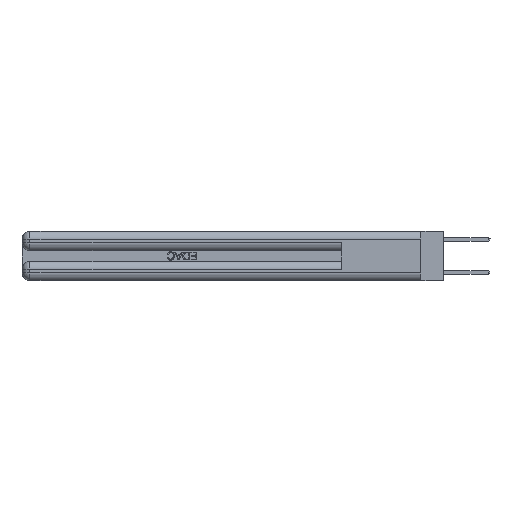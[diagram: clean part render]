
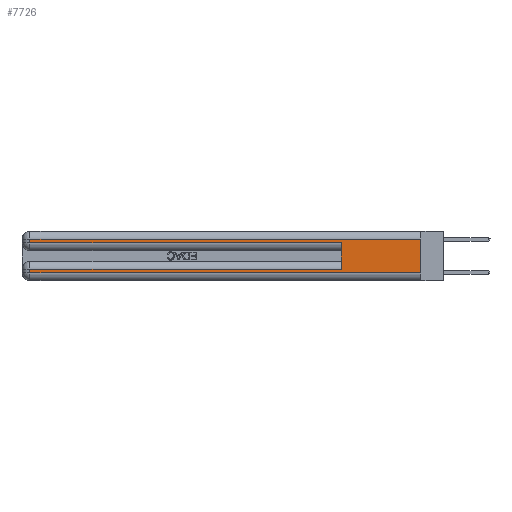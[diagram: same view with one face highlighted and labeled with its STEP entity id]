
A CAD part, left-side view. The second image highlights one B-rep face of the part: STEP entity #7726.
In plain terms, the highlighted planar face has unit normal (-1, 0, 0).
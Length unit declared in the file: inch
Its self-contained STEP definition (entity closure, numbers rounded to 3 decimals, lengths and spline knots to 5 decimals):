
#483 = DIRECTION ( 'NONE',  ( 1., 0., 0. ) ) ;
#1186 = PLANE ( 'NONE',  #19913 ) ;
#1325 = CARTESIAN_POINT ( 'NONE',  ( 0., 0., 0.31 ) ) ;
#2356 = LINE ( 'NONE', #18788, #3348 ) ;
#3005 = LINE ( 'NONE', #22045, #14640 ) ;
#3050 = LINE ( 'NONE', #23939, #21876 ) ;
#3135 = CARTESIAN_POINT ( 'NONE',  ( 0., 0.6, 0.285 ) ) ;
#3348 = VECTOR ( 'NONE', #11640, 39.37008 ) ;
#4142 = DIRECTION ( 'NONE',  ( 0., 0., -1. ) ) ;
#4411 = CARTESIAN_POINT ( 'NONE',  ( 0., 0., 0.37 ) ) ;
#4921 = ORIENTED_EDGE ( 'NONE', *, *, #17834, .T. ) ;
#5814 = VECTOR ( 'NONE', #25473, 39.37008 ) ;
#5973 = ORIENTED_EDGE ( 'NONE', *, *, #6416, .T. ) ;
#6234 = VECTOR ( 'NONE', #20308, 39.37008 ) ;
#6296 = CARTESIAN_POINT ( 'NONE',  ( 0., 2.94, 0.37 ) ) ;
#6416 = EDGE_CURVE ( 'NONE', #10710, #29371, #3005, .T. ) ;
#6460 = VERTEX_POINT ( 'NONE', #1325 ) ;
#7179 = CARTESIAN_POINT ( 'NONE',  ( 0., 0., 0.285 ) ) ;
#7595 = EDGE_CURVE ( 'NONE', #6460, #29371, #25033, .T. ) ;
#7726 = ADVANCED_FACE ( 'NONE', ( #14179 ), #1186, .F. ) ;
#8183 = CARTESIAN_POINT ( 'NONE',  ( 0., 2.94, 0.06 ) ) ;
#8397 = ORIENTED_EDGE ( 'NONE', *, *, #13000, .T. ) ;
#9335 = ORIENTED_EDGE ( 'NONE', *, *, #21855, .T. ) ;
#9799 = ORIENTED_EDGE ( 'NONE', *, *, #25341, .T. ) ;
#10225 = VERTEX_POINT ( 'NONE', #24566 ) ;
#10710 = VERTEX_POINT ( 'NONE', #8183 ) ;
#11241 = EDGE_CURVE ( 'NONE', #28706, #28387, #23354, .T. ) ;
#11640 = DIRECTION ( 'NONE',  ( 0., 1., 0. ) ) ;
#12295 = DIRECTION ( 'NONE',  ( 0., -1., 0. ) ) ;
#12493 = DIRECTION ( 'NONE',  ( 0., 0., 1. ) ) ;
#13000 = EDGE_CURVE ( 'NONE', #21127, #28706, #13157, .T. ) ;
#13157 = LINE ( 'NONE', #6296, #6234 ) ;
#13592 = EDGE_CURVE ( 'NONE', #24316, #28387, #3050, .T. ) ;
#14179 = FACE_OUTER_BOUND ( 'NONE', #17587, .T. ) ;
#14640 = VECTOR ( 'NONE', #12295, 39.37008 ) ;
#15031 = CARTESIAN_POINT ( 'NONE',  ( 0., 0., 0.085 ) ) ;
#16512 = CARTESIAN_POINT ( 'NONE',  ( 0., 2.94, 0.285 ) ) ;
#17587 = EDGE_LOOP ( 'NONE', ( #24046, #4921, #8397, #23573, #21399, #9799, #9335, #5973 ) ) ;
#17834 = EDGE_CURVE ( 'NONE', #6460, #21127, #2356, .T. ) ;
#17911 = VECTOR ( 'NONE', #24504, 39.37008 ) ;
#18309 = CARTESIAN_POINT ( 'NONE',  ( 0., 2.94, 0.37 ) ) ;
#18788 = CARTESIAN_POINT ( 'NONE',  ( 0., 0., 0.31 ) ) ;
#19913 = AXIS2_PLACEMENT_3D ( 'NONE', #25780, #483, #23935 ) ;
#20308 = DIRECTION ( 'NONE',  ( 0., 0., -1. ) ) ;
#20597 = DIRECTION ( 'NONE',  ( 0., -1., 0. ) ) ;
#21127 = VERTEX_POINT ( 'NONE', #28053 ) ;
#21399 = ORIENTED_EDGE ( 'NONE', *, *, #13592, .F. ) ;
#21855 = EDGE_CURVE ( 'NONE', #10225, #10710, #25355, .T. ) ;
#21876 = VECTOR ( 'NONE', #12493, 39.37008 ) ;
#22045 = CARTESIAN_POINT ( 'NONE',  ( 0., 0., 0.06 ) ) ;
#23354 = LINE ( 'NONE', #7179, #24624 ) ;
#23573 = ORIENTED_EDGE ( 'NONE', *, *, #11241, .T. ) ;
#23935 = DIRECTION ( 'NONE',  ( 0., 0., -1. ) ) ;
#23939 = CARTESIAN_POINT ( 'NONE',  ( 0., 0.6, 0.145 ) ) ;
#24046 = ORIENTED_EDGE ( 'NONE', *, *, #7595, .F. ) ;
#24049 = CARTESIAN_POINT ( 'NONE',  ( 0., 0.6, 0.085 ) ) ;
#24316 = VERTEX_POINT ( 'NONE', #24049 ) ;
#24504 = DIRECTION ( 'NONE',  ( 0., 1., 0. ) ) ;
#24566 = CARTESIAN_POINT ( 'NONE',  ( 0., 2.94, 0.085 ) ) ;
#24624 = VECTOR ( 'NONE', #20597, 39.37008 ) ;
#24652 = LINE ( 'NONE', #15031, #17911 ) ;
#25033 = LINE ( 'NONE', #4411, #5814 ) ;
#25341 = EDGE_CURVE ( 'NONE', #24316, #10225, #24652, .T. ) ;
#25355 = LINE ( 'NONE', #18309, #26477 ) ;
#25473 = DIRECTION ( 'NONE',  ( 0., 0., -1. ) ) ;
#25780 = CARTESIAN_POINT ( 'NONE',  ( 0., 0., 0.37 ) ) ;
#26477 = VECTOR ( 'NONE', #4142, 39.37008 ) ;
#26693 = CARTESIAN_POINT ( 'NONE',  ( 0., 0., 0.06 ) ) ;
#28053 = CARTESIAN_POINT ( 'NONE',  ( 0., 2.94, 0.31 ) ) ;
#28387 = VERTEX_POINT ( 'NONE', #3135 ) ;
#28706 = VERTEX_POINT ( 'NONE', #16512 ) ;
#29371 = VERTEX_POINT ( 'NONE', #26693 ) ;
